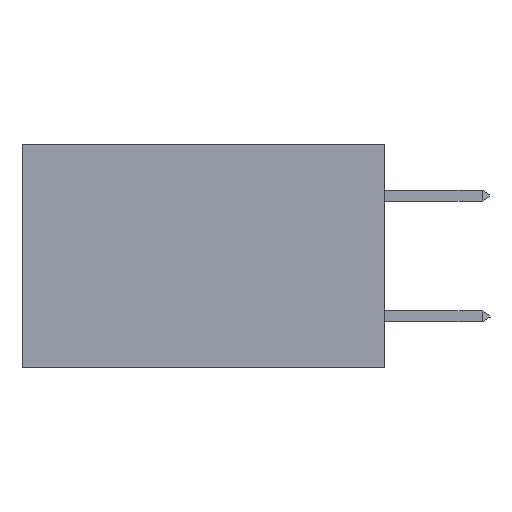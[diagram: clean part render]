
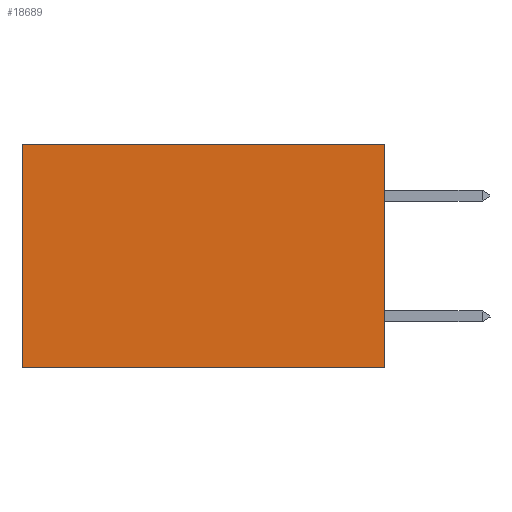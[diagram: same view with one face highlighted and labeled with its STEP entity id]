
A CAD part, left-side view. The second image highlights one B-rep face of the part: STEP entity #18689.
In plain terms, the highlighted planar face has unit normal (-1, 0, 0).
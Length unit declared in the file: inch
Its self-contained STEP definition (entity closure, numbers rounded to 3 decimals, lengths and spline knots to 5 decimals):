
#750 = ORIENTED_EDGE ( 'NONE', *, *, #20745, .F. ) ;
#1042 = VECTOR ( 'NONE', #7013, 39.37008 ) ;
#1246 = CARTESIAN_POINT ( 'NONE',  ( 0.2875, 0., -0.37 ) ) ;
#2906 = PLANE ( 'NONE',  #20445 ) ;
#3244 = LINE ( 'NONE', #8876, #20770 ) ;
#5642 = VECTOR ( 'NONE', #30864, 39.37008 ) ;
#7013 = DIRECTION ( 'NONE',  ( 0., 0., -1. ) ) ;
#7168 = EDGE_CURVE ( 'NONE', #22458, #21797, #3244, .T. ) ;
#7404 = LINE ( 'NONE', #16375, #1042 ) ;
#8876 = CARTESIAN_POINT ( 'NONE',  ( 0.2875, 0., -0.37 ) ) ;
#9813 = ORIENTED_EDGE ( 'NONE', *, *, #28771, .T. ) ;
#9834 = ORIENTED_EDGE ( 'NONE', *, *, #16851, .T. ) ;
#10063 = CARTESIAN_POINT ( 'NONE',  ( 0.2875, 0., 0. ) ) ;
#11426 = ORIENTED_EDGE ( 'NONE', *, *, #7168, .F. ) ;
#11849 = CARTESIAN_POINT ( 'NONE',  ( 0.2875, 0., 0. ) ) ;
#11978 = LINE ( 'NONE', #19401, #5642 ) ;
#12359 = FACE_OUTER_BOUND ( 'NONE', #15184, .T. ) ;
#13064 = LINE ( 'NONE', #28309, #13840 ) ;
#13840 = VECTOR ( 'NONE', #19058, 39.37008 ) ;
#15184 = EDGE_LOOP ( 'NONE', ( #9813, #11426, #750, #9834 ) ) ;
#16375 = CARTESIAN_POINT ( 'NONE',  ( 0.2875, 0., 0. ) ) ;
#16850 = DIRECTION ( 'NONE',  ( 0., 0., -1. ) ) ;
#16851 = EDGE_CURVE ( 'NONE', #23400, #24728, #11978, .T. ) ;
#18689 = ADVANCED_FACE ( 'NONE', ( #12359 ), #2906, .F. ) ;
#19058 = DIRECTION ( 'NONE',  ( 0., 0., -1. ) ) ;
#19401 = CARTESIAN_POINT ( 'NONE',  ( 0.2875, 0., 0. ) ) ;
#20036 = DIRECTION ( 'NONE',  ( 0., 1., 0. ) ) ;
#20445 = AXIS2_PLACEMENT_3D ( 'NONE', #10063, #28915, #16850 ) ;
#20606 = CARTESIAN_POINT ( 'NONE',  ( 0.2875, 0.6, -0.37 ) ) ;
#20745 = EDGE_CURVE ( 'NONE', #23400, #22458, #7404, .T. ) ;
#20770 = VECTOR ( 'NONE', #20036, 39.37008 ) ;
#21797 = VERTEX_POINT ( 'NONE', #20606 ) ;
#22458 = VERTEX_POINT ( 'NONE', #1246 ) ;
#23400 = VERTEX_POINT ( 'NONE', #11849 ) ;
#24304 = CARTESIAN_POINT ( 'NONE',  ( 0.2875, 0.6, 0. ) ) ;
#24728 = VERTEX_POINT ( 'NONE', #24304 ) ;
#28309 = CARTESIAN_POINT ( 'NONE',  ( 0.2875, 0.6, 0. ) ) ;
#28771 = EDGE_CURVE ( 'NONE', #24728, #21797, #13064, .T. ) ;
#28915 = DIRECTION ( 'NONE',  ( 1., 0., 0. ) ) ;
#30864 = DIRECTION ( 'NONE',  ( 0., 1., 0. ) ) ;
